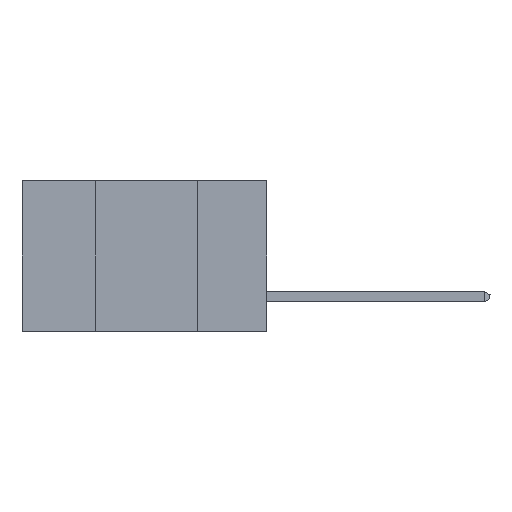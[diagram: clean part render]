
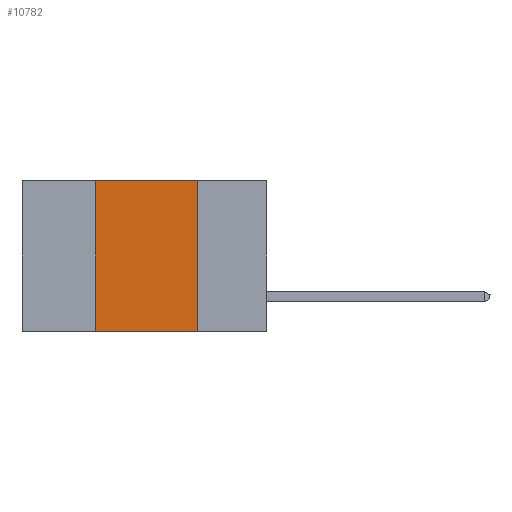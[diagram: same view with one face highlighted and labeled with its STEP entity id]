
A CAD part, left-side view. The second image highlights one B-rep face of the part: STEP entity #10782.
In plain terms, the highlighted planar face has unit normal (-1, 0, 0).
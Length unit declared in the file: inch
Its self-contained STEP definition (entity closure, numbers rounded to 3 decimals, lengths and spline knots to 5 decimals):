
#89 = DIRECTION ( 'NONE',  ( 0., 0., 1. ) ) ;
#861 = EDGE_CURVE ( 'NONE', #6834, #9877, #2203, .T. ) ;
#947 = VERTEX_POINT ( 'NONE', #10361 ) ;
#967 = DIRECTION ( 'NONE',  ( 0., -1., 0. ) ) ;
#1174 = ORIENTED_EDGE ( 'NONE', *, *, #861, .F. ) ;
#2203 = LINE ( 'NONE', #11673, #12941 ) ;
#2612 = PLANE ( 'NONE',  #8617 ) ;
#2659 = ORIENTED_EDGE ( 'NONE', *, *, #6853, .F. ) ;
#3012 = EDGE_CURVE ( 'NONE', #3770, #947, #4158, .T. ) ;
#3520 = EDGE_CURVE ( 'NONE', #3770, #9877, #3574, .T. ) ;
#3574 = LINE ( 'NONE', #5461, #10660 ) ;
#3770 = VERTEX_POINT ( 'NONE', #8276 ) ;
#3870 = CARTESIAN_POINT ( 'NONE',  ( 0., 0.6, 0. ) ) ;
#4158 = LINE ( 'NONE', #6305, #8991 ) ;
#4632 = EDGE_LOOP ( 'NONE', ( #1174, #2659, #8788, #7714 ) ) ;
#5461 = CARTESIAN_POINT ( 'NONE',  ( 0., 0.6, -0.37 ) ) ;
#6144 = LINE ( 'NONE', #11474, #12655 ) ;
#6305 = CARTESIAN_POINT ( 'NONE',  ( 0., 0.42, 0. ) ) ;
#6834 = VERTEX_POINT ( 'NONE', #12581 ) ;
#6853 = EDGE_CURVE ( 'NONE', #947, #6834, #6144, .T. ) ;
#7714 = ORIENTED_EDGE ( 'NONE', *, *, #3520, .T. ) ;
#8276 = CARTESIAN_POINT ( 'NONE',  ( 0., 0.42, -0.37 ) ) ;
#8361 = DIRECTION ( 'NONE',  ( 0., 0., -1. ) ) ;
#8617 = AXIS2_PLACEMENT_3D ( 'NONE', #3870, #11197, #12154 ) ;
#8788 = ORIENTED_EDGE ( 'NONE', *, *, #3012, .F. ) ;
#8991 = VECTOR ( 'NONE', #89, 39.37008 ) ;
#9877 = VERTEX_POINT ( 'NONE', #11870 ) ;
#10361 = CARTESIAN_POINT ( 'NONE',  ( 0., 0.42, 0. ) ) ;
#10660 = VECTOR ( 'NONE', #11743, 39.37008 ) ;
#10782 = ADVANCED_FACE ( 'NONE', ( #11133 ), #2612, .F. ) ;
#11133 = FACE_OUTER_BOUND ( 'NONE', #4632, .T. ) ;
#11197 = DIRECTION ( 'NONE',  ( 1., 0., 0. ) ) ;
#11474 = CARTESIAN_POINT ( 'NONE',  ( 0., 0.6, 0. ) ) ;
#11673 = CARTESIAN_POINT ( 'NONE',  ( 0., 0.17, 0. ) ) ;
#11743 = DIRECTION ( 'NONE',  ( 0., -1., 0. ) ) ;
#11870 = CARTESIAN_POINT ( 'NONE',  ( 0., 0.17, -0.37 ) ) ;
#12154 = DIRECTION ( 'NONE',  ( 0., 0., -1. ) ) ;
#12581 = CARTESIAN_POINT ( 'NONE',  ( 0., 0.17, 0. ) ) ;
#12655 = VECTOR ( 'NONE', #967, 39.37008 ) ;
#12941 = VECTOR ( 'NONE', #8361, 39.37008 ) ;
